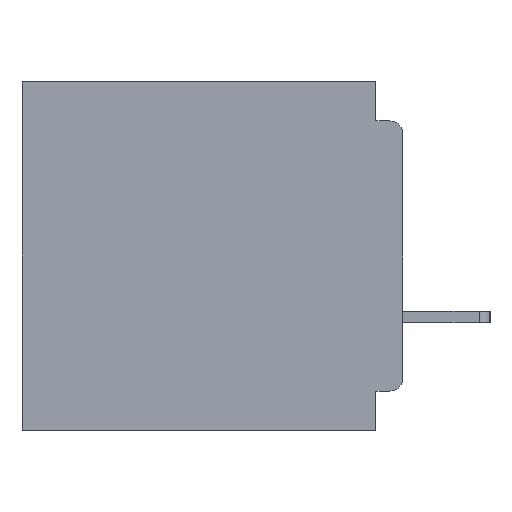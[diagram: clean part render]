
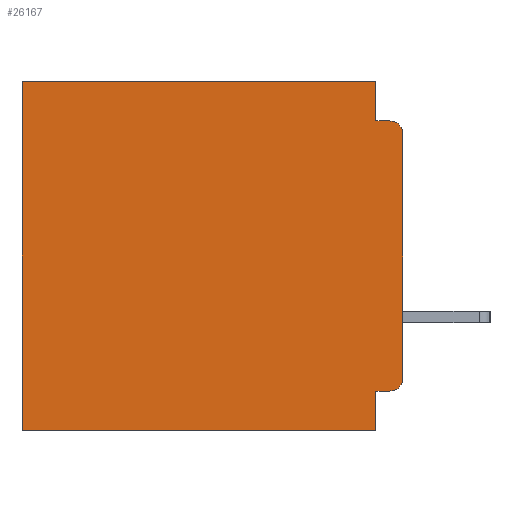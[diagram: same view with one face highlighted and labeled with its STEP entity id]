
A CAD part, left-side view. The second image highlights one B-rep face of the part: STEP entity #26167.
In plain terms, the highlighted planar face has unit normal (-1, 0, 0).
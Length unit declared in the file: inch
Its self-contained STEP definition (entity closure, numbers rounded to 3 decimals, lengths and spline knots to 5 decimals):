
#40 = CARTESIAN_POINT ( 'NONE',  ( 0.3, 0., -0.06 ) ) ;
#636 = DIRECTION ( 'NONE',  ( 0., 0., -1. ) ) ;
#641 = VERTEX_POINT ( 'NONE', #40 ) ;
#1733 = VECTOR ( 'NONE', #37492, 39.37008 ) ;
#1814 = CARTESIAN_POINT ( 'NONE',  ( 0.3, 0.015, -0.045 ) ) ;
#2067 = CARTESIAN_POINT ( 'NONE',  ( 0.3, 0., -0.34 ) ) ;
#2536 = DIRECTION ( 'NONE',  ( 0., 0., -1. ) ) ;
#3219 = VECTOR ( 'NONE', #13632, 39.37008 ) ;
#3400 = CARTESIAN_POINT ( 'NONE',  ( 0.3, 0., -0.4 ) ) ;
#3976 = VERTEX_POINT ( 'NONE', #13093 ) ;
#4629 = DIRECTION ( 'NONE',  ( -1., 0., 0. ) ) ;
#5101 = EDGE_CURVE ( 'NONE', #33419, #36193, #35451, .T. ) ;
#5235 = CARTESIAN_POINT ( 'NONE',  ( 0.3, 0., -0.355 ) ) ;
#5382 = DIRECTION ( 'NONE',  ( 0., 0., -1. ) ) ;
#5475 = CARTESIAN_POINT ( 'NONE',  ( 0.3, 0., 0. ) ) ;
#5827 = VERTEX_POINT ( 'NONE', #30900 ) ;
#6287 = VERTEX_POINT ( 'NONE', #21981 ) ;
#6300 = CARTESIAN_POINT ( 'NONE',  ( 0.3, 0.437, 0. ) ) ;
#7184 = LINE ( 'NONE', #13594, #27375 ) ;
#7520 = PLANE ( 'NONE',  #50343 ) ;
#8473 = EDGE_CURVE ( 'NONE', #6287, #33419, #35040, .T. ) ;
#9313 = LINE ( 'NONE', #24035, #40211 ) ;
#11602 = DIRECTION ( 'NONE',  ( 0., 0., -1. ) ) ;
#11785 = ORIENTED_EDGE ( 'NONE', *, *, #41955, .F. ) ;
#12372 = DIRECTION ( 'NONE',  ( -1., 0., 0. ) ) ;
#13093 = CARTESIAN_POINT ( 'NONE',  ( 0.3, 0.031, -0.045 ) ) ;
#13594 = CARTESIAN_POINT ( 'NONE',  ( 0.3, 0.031, 0. ) ) ;
#13631 = EDGE_CURVE ( 'NONE', #3976, #49122, #9313, .T. ) ;
#13632 = DIRECTION ( 'NONE',  ( 0., 1., 0. ) ) ;
#13661 = VECTOR ( 'NONE', #2536, 39.37008 ) ;
#13684 = DIRECTION ( 'NONE',  ( 0., 1., 0. ) ) ;
#14899 = ORIENTED_EDGE ( 'NONE', *, *, #8473, .F. ) ;
#15016 = EDGE_CURVE ( 'NONE', #5827, #33882, #16483, .T. ) ;
#15604 = EDGE_CURVE ( 'NONE', #48406, #6287, #31433, .T. ) ;
#15689 = ORIENTED_EDGE ( 'NONE', *, *, #44513, .T. ) ;
#16483 = LINE ( 'NONE', #5475, #36573 ) ;
#18091 = CIRCLE ( 'NONE', #31848, 0.015 ) ;
#21107 = CARTESIAN_POINT ( 'NONE',  ( 0.3, 0., -0.4 ) ) ;
#21252 = EDGE_CURVE ( 'NONE', #641, #23429, #40543, .T. ) ;
#21703 = ORIENTED_EDGE ( 'NONE', *, *, #5101, .F. ) ;
#21981 = CARTESIAN_POINT ( 'NONE',  ( 0.3, 0.031, -0.355 ) ) ;
#22014 = ORIENTED_EDGE ( 'NONE', *, *, #15016, .T. ) ;
#22808 = CARTESIAN_POINT ( 'NONE',  ( 0.3, 0.437, -0.4 ) ) ;
#22899 = ORIENTED_EDGE ( 'NONE', *, *, #21252, .F. ) ;
#23429 = VERTEX_POINT ( 'NONE', #2067 ) ;
#24035 = CARTESIAN_POINT ( 'NONE',  ( 0.3, 0., -0.045 ) ) ;
#25121 = ORIENTED_EDGE ( 'NONE', *, *, #13631, .F. ) ;
#26167 = ADVANCED_FACE ( 'NONE', ( #40058 ), #7520, .F. ) ;
#26803 = AXIS2_PLACEMENT_3D ( 'NONE', #36452, #12372, #40497 ) ;
#27077 = VECTOR ( 'NONE', #41979, 39.37008 ) ;
#27361 = ORIENTED_EDGE ( 'NONE', *, *, #41066, .T. ) ;
#27375 = VECTOR ( 'NONE', #5382, 39.37008 ) ;
#28751 = CARTESIAN_POINT ( 'NONE',  ( 0.3, 0.015, -0.06 ) ) ;
#30900 = CARTESIAN_POINT ( 'NONE',  ( 0.3, 0.031, 0. ) ) ;
#31433 = LINE ( 'NONE', #5235, #1733 ) ;
#31848 = AXIS2_PLACEMENT_3D ( 'NONE', #28751, #4629, #32859 ) ;
#32670 = EDGE_LOOP ( 'NONE', ( #22899, #27361, #25121, #11785, #22014, #15689, #21703, #14899, #51085, #46809 ) ) ;
#32859 = DIRECTION ( 'NONE',  ( 0., 0., -1. ) ) ;
#33419 = VERTEX_POINT ( 'NONE', #39831 ) ;
#33657 = CARTESIAN_POINT ( 'NONE',  ( 0.3, 0., -0.4 ) ) ;
#33882 = VERTEX_POINT ( 'NONE', #6300 ) ;
#35040 = LINE ( 'NONE', #50817, #13661 ) ;
#35451 = LINE ( 'NONE', #33657, #3219 ) ;
#35724 = DIRECTION ( 'NONE',  ( 1., 0., 0. ) ) ;
#36122 = DIRECTION ( 'NONE',  ( 0., -1., 0. ) ) ;
#36193 = VERTEX_POINT ( 'NONE', #22808 ) ;
#36452 = CARTESIAN_POINT ( 'NONE',  ( 0.3, 0.015, -0.34 ) ) ;
#36573 = VECTOR ( 'NONE', #13684, 39.37008 ) ;
#37492 = DIRECTION ( 'NONE',  ( 0., 1., 0. ) ) ;
#39831 = CARTESIAN_POINT ( 'NONE',  ( 0.3, 0.031, -0.4 ) ) ;
#40058 = FACE_OUTER_BOUND ( 'NONE', #32670, .T. ) ;
#40211 = VECTOR ( 'NONE', #36122, 39.37008 ) ;
#40434 = EDGE_CURVE ( 'NONE', #48406, #23429, #49552, .T. ) ;
#40497 = DIRECTION ( 'NONE',  ( 0., 0., -1. ) ) ;
#40543 = LINE ( 'NONE', #21107, #51201 ) ;
#41066 = EDGE_CURVE ( 'NONE', #641, #49122, #18091, .T. ) ;
#41278 = CARTESIAN_POINT ( 'NONE',  ( 0.3, 0.015, -0.355 ) ) ;
#41955 = EDGE_CURVE ( 'NONE', #5827, #3976, #7184, .T. ) ;
#41979 = DIRECTION ( 'NONE',  ( 0., 0., -1. ) ) ;
#44513 = EDGE_CURVE ( 'NONE', #33882, #36193, #48473, .T. ) ;
#45839 = CARTESIAN_POINT ( 'NONE',  ( 0.3, 0.437, -0.4 ) ) ;
#46809 = ORIENTED_EDGE ( 'NONE', *, *, #40434, .T. ) ;
#48406 = VERTEX_POINT ( 'NONE', #41278 ) ;
#48473 = LINE ( 'NONE', #45839, #27077 ) ;
#49122 = VERTEX_POINT ( 'NONE', #1814 ) ;
#49552 = CIRCLE ( 'NONE', #26803, 0.015 ) ;
#50343 = AXIS2_PLACEMENT_3D ( 'NONE', #3400, #35724, #11602 ) ;
#50817 = CARTESIAN_POINT ( 'NONE',  ( 0.3, 0.031, -0.4 ) ) ;
#51085 = ORIENTED_EDGE ( 'NONE', *, *, #15604, .F. ) ;
#51201 = VECTOR ( 'NONE', #636, 39.37008 ) ;
